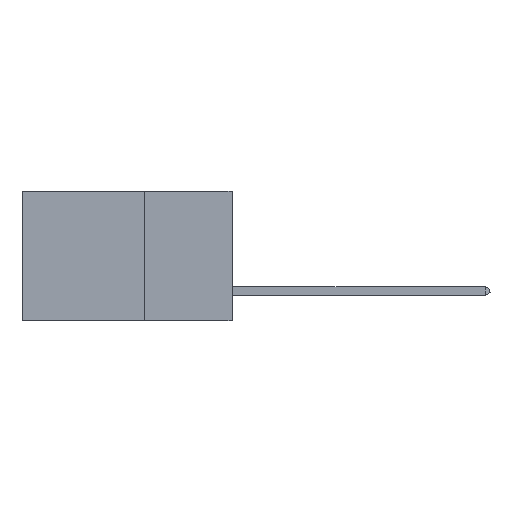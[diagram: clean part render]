
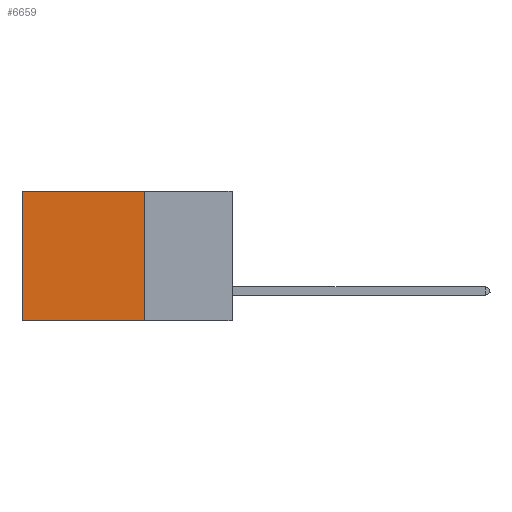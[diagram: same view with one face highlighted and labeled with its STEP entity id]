
A CAD part, left-side view. The second image highlights one B-rep face of the part: STEP entity #6659.
In plain terms, the highlighted planar face has unit normal (-1, 0, 0).
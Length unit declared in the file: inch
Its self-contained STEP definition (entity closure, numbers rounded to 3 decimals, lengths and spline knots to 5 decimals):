
#806 = CARTESIAN_POINT ( 'NONE',  ( 0.2875, 0.25, -0.37 ) ) ;
#2186 = VECTOR ( 'NONE', #9989, 39.37008 ) ;
#2981 = VERTEX_POINT ( 'NONE', #17558 ) ;
#2984 = VERTEX_POINT ( 'NONE', #806 ) ;
#4109 = DIRECTION ( 'NONE',  ( 0., 0., -1. ) ) ;
#4700 = DIRECTION ( 'NONE',  ( 1., 0., 0. ) ) ;
#5538 = DIRECTION ( 'NONE',  ( 0., 1., 0. ) ) ;
#6305 = EDGE_CURVE ( 'NONE', #2981, #23364, #14273, .T. ) ;
#6659 = ADVANCED_FACE ( 'NONE', ( #21217 ), #10502, .F. ) ;
#7157 = CARTESIAN_POINT ( 'NONE',  ( 0.2875, 0.25, 0. ) ) ;
#7585 = CARTESIAN_POINT ( 'NONE',  ( 0.2875, 0.25, -0.37 ) ) ;
#7987 = CARTESIAN_POINT ( 'NONE',  ( 0.2875, 0.6, 0. ) ) ;
#8573 = CARTESIAN_POINT ( 'NONE',  ( 0.2875, 0.25, 0. ) ) ;
#8752 = ORIENTED_EDGE ( 'NONE', *, *, #17026, .F. ) ;
#9989 = DIRECTION ( 'NONE',  ( 0., 0., -1. ) ) ;
#10029 = CARTESIAN_POINT ( 'NONE',  ( 0.2875, 0.6, 0. ) ) ;
#10502 = PLANE ( 'NONE',  #20916 ) ;
#11069 = VECTOR ( 'NONE', #5538, 39.37008 ) ;
#11829 = LINE ( 'NONE', #7987, #13444 ) ;
#12010 = ORIENTED_EDGE ( 'NONE', *, *, #14858, .T. ) ;
#13444 = VECTOR ( 'NONE', #4109, 39.37008 ) ;
#13575 = CARTESIAN_POINT ( 'NONE',  ( 0.2875, 0.25, 0. ) ) ;
#14083 = DIRECTION ( 'NONE',  ( 0., 0., -1. ) ) ;
#14133 = EDGE_LOOP ( 'NONE', ( #12010, #21479, #8752, #15893 ) ) ;
#14273 = LINE ( 'NONE', #7157, #22048 ) ;
#14858 = EDGE_CURVE ( 'NONE', #23364, #15772, #11829, .T. ) ;
#15772 = VERTEX_POINT ( 'NONE', #23176 ) ;
#15893 = ORIENTED_EDGE ( 'NONE', *, *, #6305, .T. ) ;
#16320 = DIRECTION ( 'NONE',  ( 0., 1., 0. ) ) ;
#17026 = EDGE_CURVE ( 'NONE', #2981, #2984, #22735, .T. ) ;
#17558 = CARTESIAN_POINT ( 'NONE',  ( 0.2875, 0.25, 0. ) ) ;
#19288 = EDGE_CURVE ( 'NONE', #2984, #15772, #22281, .T. ) ;
#20916 = AXIS2_PLACEMENT_3D ( 'NONE', #8573, #4700, #14083 ) ;
#21217 = FACE_OUTER_BOUND ( 'NONE', #14133, .T. ) ;
#21479 = ORIENTED_EDGE ( 'NONE', *, *, #19288, .F. ) ;
#22048 = VECTOR ( 'NONE', #16320, 39.37008 ) ;
#22281 = LINE ( 'NONE', #7585, #11069 ) ;
#22735 = LINE ( 'NONE', #13575, #2186 ) ;
#23176 = CARTESIAN_POINT ( 'NONE',  ( 0.2875, 0.6, -0.37 ) ) ;
#23364 = VERTEX_POINT ( 'NONE', #10029 ) ;
